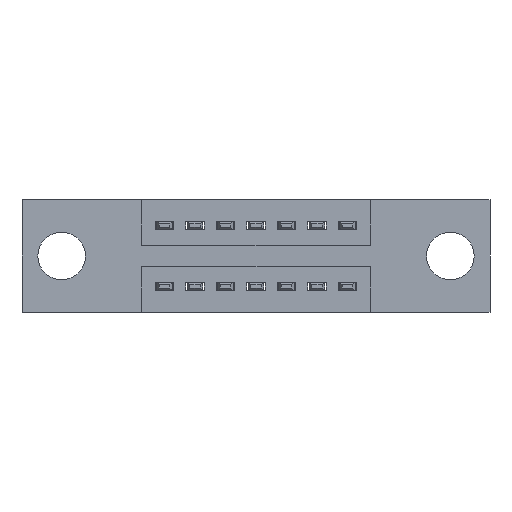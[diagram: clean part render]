
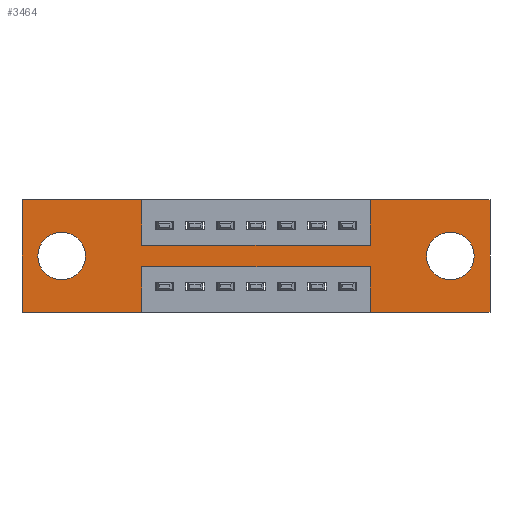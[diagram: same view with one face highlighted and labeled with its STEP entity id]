
A CAD part, front view. The second image highlights one B-rep face of the part: STEP entity #3464.
In plain terms, the highlighted planar face has unit normal (0, -1, 0).
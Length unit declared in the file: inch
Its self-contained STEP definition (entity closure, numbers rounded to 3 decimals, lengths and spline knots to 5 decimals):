
#102 = LINE ( 'NONE', #6496, #3637 ) ;
#240 = ORIENTED_EDGE ( 'NONE', *, *, #6238, .T. ) ;
#433 = CARTESIAN_POINT ( 'NONE',  ( 1.535, 0., 0. ) ) ;
#499 = EDGE_CURVE ( 'NONE', #3250, #2320, #7963, .T. ) ;
#530 = VERTEX_POINT ( 'NONE', #4773 ) ;
#573 = DIRECTION ( 'NONE',  ( 0., 1., 0. ) ) ;
#645 = CARTESIAN_POINT ( 'NONE',  ( 0., 0., -0.37 ) ) ;
#693 = ORIENTED_EDGE ( 'NONE', *, *, #1071, .F. ) ;
#815 = CARTESIAN_POINT ( 'NONE',  ( 1.535, 0., 0. ) ) ;
#839 = LINE ( 'NONE', #5701, #4201 ) ;
#951 = VECTOR ( 'NONE', #8858, 39.37008 ) ;
#953 = LINE ( 'NONE', #2516, #1004 ) ;
#1004 = VECTOR ( 'NONE', #5005, 39.37008 ) ;
#1071 = EDGE_CURVE ( 'NONE', #9457, #1078, #839, .T. ) ;
#1078 = VERTEX_POINT ( 'NONE', #6451 ) ;
#1094 = DIRECTION ( 'NONE',  ( 0., 0., 1. ) ) ;
#1287 = VERTEX_POINT ( 'NONE', #5912 ) ;
#1361 = AXIS2_PLACEMENT_3D ( 'NONE', #7787, #573, #3607 ) ;
#1465 = VERTEX_POINT ( 'NONE', #2401 ) ;
#1709 = EDGE_CURVE ( 'NONE', #1287, #2211, #2067, .T. ) ;
#1719 = AXIS2_PLACEMENT_3D ( 'NONE', #6663, #4917, #9910 ) ;
#1809 = VECTOR ( 'NONE', #9220, 39.37008 ) ;
#1819 = ORIENTED_EDGE ( 'NONE', *, *, #499, .F. ) ;
#1907 = ORIENTED_EDGE ( 'NONE', *, *, #7766, .F. ) ;
#1965 = DIRECTION ( 'NONE',  ( 0., 0., 1. ) ) ;
#1994 = ORIENTED_EDGE ( 'NONE', *, *, #2179, .F. ) ;
#2067 = LINE ( 'NONE', #6748, #8802 ) ;
#2179 = EDGE_CURVE ( 'NONE', #1465, #530, #3560, .T. ) ;
#2211 = VERTEX_POINT ( 'NONE', #7625 ) ;
#2268 = CARTESIAN_POINT ( 'NONE',  ( 1.405, 0., -0.263 ) ) ;
#2304 = EDGE_CURVE ( 'NONE', #9326, #5478, #9652, .T. ) ;
#2320 = VERTEX_POINT ( 'NONE', #7899 ) ;
#2352 = ORIENTED_EDGE ( 'NONE', *, *, #10429, .T. ) ;
#2386 = DIRECTION ( 'NONE',  ( 0., 0., -1. ) ) ;
#2401 = CARTESIAN_POINT ( 'NONE',  ( 0., 0., 0. ) ) ;
#2409 = EDGE_CURVE ( 'NONE', #9367, #4987, #10345, .T. ) ;
#2419 = DIRECTION ( 'NONE',  ( -1., 0., 0. ) ) ;
#2483 = ORIENTED_EDGE ( 'NONE', *, *, #1709, .F. ) ;
#2516 = CARTESIAN_POINT ( 'NONE',  ( 0., 0., 0. ) ) ;
#2690 = DIRECTION ( 'NONE',  ( 0., -1., 0. ) ) ;
#2788 = ORIENTED_EDGE ( 'NONE', *, *, #9125, .F. ) ;
#2797 = DIRECTION ( 'NONE',  ( 0., 0., -1. ) ) ;
#3108 = ORIENTED_EDGE ( 'NONE', *, *, #2409, .T. ) ;
#3250 = VERTEX_POINT ( 'NONE', #4840 ) ;
#3322 = VERTEX_POINT ( 'NONE', #433 ) ;
#3384 = EDGE_CURVE ( 'NONE', #4987, #9367, #4034, .T. ) ;
#3464 = ADVANCED_FACE ( 'NONE', ( #4462, #9203, #6687 ), #5891, .T. ) ;
#3549 = VECTOR ( 'NONE', #9284, 39.37008 ) ;
#3560 = LINE ( 'NONE', #9234, #3549 ) ;
#3607 = DIRECTION ( 'NONE',  ( 0., 0., 1. ) ) ;
#3637 = VECTOR ( 'NONE', #8201, 39.37008 ) ;
#3849 = CARTESIAN_POINT ( 'NONE',  ( 1.1425, 0., -0.37 ) ) ;
#4034 = CIRCLE ( 'NONE', #6555, 0.078 ) ;
#4201 = VECTOR ( 'NONE', #8101, 39.37008 ) ;
#4323 = ORIENTED_EDGE ( 'NONE', *, *, #7859, .F. ) ;
#4358 = CARTESIAN_POINT ( 'NONE',  ( 0., 0., -0.37 ) ) ;
#4414 = DIRECTION ( 'NONE',  ( 0., 1., 0. ) ) ;
#4426 = CARTESIAN_POINT ( 'NONE',  ( 0.13, 0., -0.185 ) ) ;
#4462 = FACE_BOUND ( 'NONE', #4902, .T. ) ;
#4491 = EDGE_LOOP ( 'NONE', ( #1907, #6309, #9338, #1819, #6813, #7499, #6248, #693, #2788, #1994, #4323, #2483 ) ) ;
#4658 = CARTESIAN_POINT ( 'NONE',  ( 0.3925, 0., -0.22 ) ) ;
#4773 = CARTESIAN_POINT ( 'NONE',  ( 0.3925, 0., 0. ) ) ;
#4775 = CARTESIAN_POINT ( 'NONE',  ( 1.1425, 0., -0.22 ) ) ;
#4840 = CARTESIAN_POINT ( 'NONE',  ( 1.535, 0., -0.37 ) ) ;
#4902 = EDGE_LOOP ( 'NONE', ( #5077, #3108 ) ) ;
#4917 = DIRECTION ( 'NONE',  ( 0., 1., 0. ) ) ;
#4987 = VERTEX_POINT ( 'NONE', #7512 ) ;
#5005 = DIRECTION ( 'NONE',  ( 1., 0., 0. ) ) ;
#5020 = CIRCLE ( 'NONE', #1361, 0.078 ) ;
#5055 = LINE ( 'NONE', #815, #8057 ) ;
#5077 = ORIENTED_EDGE ( 'NONE', *, *, #3384, .T. ) ;
#5270 = CARTESIAN_POINT ( 'NONE',  ( 0., 0., 0. ) ) ;
#5406 = LINE ( 'NONE', #9346, #8771 ) ;
#5478 = VERTEX_POINT ( 'NONE', #10434 ) ;
#5701 = CARTESIAN_POINT ( 'NONE',  ( 0.3925, 0., -0.15 ) ) ;
#5879 = AXIS2_PLACEMENT_3D ( 'NONE', #4358, #2690, #7688 ) ;
#5891 = PLANE ( 'NONE',  #5879 ) ;
#5908 = CARTESIAN_POINT ( 'NONE',  ( 0.13, 0., -0.263 ) ) ;
#5912 = CARTESIAN_POINT ( 'NONE',  ( 0.3925, 0., -0.37 ) ) ;
#6037 = DIRECTION ( 'NONE',  ( 0., 0., -1. ) ) ;
#6238 = EDGE_CURVE ( 'NONE', #6681, #7256, #5020, .T. ) ;
#6248 = ORIENTED_EDGE ( 'NONE', *, *, #7527, .F. ) ;
#6309 = ORIENTED_EDGE ( 'NONE', *, *, #2304, .F. ) ;
#6451 = CARTESIAN_POINT ( 'NONE',  ( 1.1425, 0., -0.15 ) ) ;
#6496 = CARTESIAN_POINT ( 'NONE',  ( 0.3925, 0., -0.37 ) ) ;
#6555 = AXIS2_PLACEMENT_3D ( 'NONE', #7535, #4414, #2797 ) ;
#6570 = CARTESIAN_POINT ( 'NONE',  ( 0.13, 0., -0.107 ) ) ;
#6663 = CARTESIAN_POINT ( 'NONE',  ( 1.405, 0., -0.185 ) ) ;
#6681 = VERTEX_POINT ( 'NONE', #5908 ) ;
#6687 = FACE_OUTER_BOUND ( 'NONE', #4491, .T. ) ;
#6748 = CARTESIAN_POINT ( 'NONE',  ( 0., 0., -0.37 ) ) ;
#6813 = ORIENTED_EDGE ( 'NONE', *, *, #8854, .F. ) ;
#6815 = LINE ( 'NONE', #5270, #1809 ) ;
#7132 = EDGE_LOOP ( 'NONE', ( #2352, #240 ) ) ;
#7256 = VERTEX_POINT ( 'NONE', #6570 ) ;
#7467 = CARTESIAN_POINT ( 'NONE',  ( 0.3925, 0., -0.15 ) ) ;
#7499 = ORIENTED_EDGE ( 'NONE', *, *, #9894, .F. ) ;
#7512 = CARTESIAN_POINT ( 'NONE',  ( 1.405, 0., -0.107 ) ) ;
#7527 = EDGE_CURVE ( 'NONE', #1078, #9092, #7953, .T. ) ;
#7535 = CARTESIAN_POINT ( 'NONE',  ( 1.405, 0., -0.185 ) ) ;
#7625 = CARTESIAN_POINT ( 'NONE',  ( 0., 0., -0.37 ) ) ;
#7688 = DIRECTION ( 'NONE',  ( 0., 0., -1. ) ) ;
#7701 = VECTOR ( 'NONE', #1094, 39.37008 ) ;
#7766 = EDGE_CURVE ( 'NONE', #5478, #1287, #102, .T. ) ;
#7787 = CARTESIAN_POINT ( 'NONE',  ( 0.13, 0., -0.185 ) ) ;
#7859 = EDGE_CURVE ( 'NONE', #2211, #1465, #6815, .T. ) ;
#7899 = CARTESIAN_POINT ( 'NONE',  ( 1.1425, 0., -0.37 ) ) ;
#7953 = LINE ( 'NONE', #9597, #951 ) ;
#7963 = LINE ( 'NONE', #645, #8252 ) ;
#8057 = VECTOR ( 'NONE', #2386, 39.37008 ) ;
#8101 = DIRECTION ( 'NONE',  ( 1., 0., 0. ) ) ;
#8201 = DIRECTION ( 'NONE',  ( 0., 0., -1. ) ) ;
#8252 = VECTOR ( 'NONE', #10379, 39.37008 ) ;
#8287 = CARTESIAN_POINT ( 'NONE',  ( 1.1425, 0., 0. ) ) ;
#8300 = AXIS2_PLACEMENT_3D ( 'NONE', #4426, #8350, #1965 ) ;
#8350 = DIRECTION ( 'NONE',  ( 0., 1., 0. ) ) ;
#8450 = VECTOR ( 'NONE', #2419, 39.37008 ) ;
#8456 = DIRECTION ( 'NONE',  ( -1., 0., 0. ) ) ;
#8771 = VECTOR ( 'NONE', #6037, 39.37008 ) ;
#8786 = EDGE_CURVE ( 'NONE', #2320, #9326, #10275, .T. ) ;
#8802 = VECTOR ( 'NONE', #8456, 39.37008 ) ;
#8825 = CIRCLE ( 'NONE', #8300, 0.078 ) ;
#8854 = EDGE_CURVE ( 'NONE', #3322, #3250, #5055, .T. ) ;
#8858 = DIRECTION ( 'NONE',  ( 0., 0., 1. ) ) ;
#9092 = VERTEX_POINT ( 'NONE', #8287 ) ;
#9125 = EDGE_CURVE ( 'NONE', #530, #9457, #5406, .T. ) ;
#9203 = FACE_BOUND ( 'NONE', #7132, .T. ) ;
#9220 = DIRECTION ( 'NONE',  ( 0., 0., 1. ) ) ;
#9234 = CARTESIAN_POINT ( 'NONE',  ( 0., 0., 0. ) ) ;
#9284 = DIRECTION ( 'NONE',  ( 1., 0., 0. ) ) ;
#9326 = VERTEX_POINT ( 'NONE', #4775 ) ;
#9338 = ORIENTED_EDGE ( 'NONE', *, *, #8786, .F. ) ;
#9346 = CARTESIAN_POINT ( 'NONE',  ( 0.3925, 0., 0. ) ) ;
#9367 = VERTEX_POINT ( 'NONE', #2268 ) ;
#9457 = VERTEX_POINT ( 'NONE', #7467 ) ;
#9597 = CARTESIAN_POINT ( 'NONE',  ( 1.1425, 0., 0. ) ) ;
#9652 = LINE ( 'NONE', #4658, #8450 ) ;
#9894 = EDGE_CURVE ( 'NONE', #9092, #3322, #953, .T. ) ;
#9910 = DIRECTION ( 'NONE',  ( 0., 0., -1. ) ) ;
#10275 = LINE ( 'NONE', #3849, #7701 ) ;
#10345 = CIRCLE ( 'NONE', #1719, 0.078 ) ;
#10379 = DIRECTION ( 'NONE',  ( -1., 0., 0. ) ) ;
#10429 = EDGE_CURVE ( 'NONE', #7256, #6681, #8825, .T. ) ;
#10434 = CARTESIAN_POINT ( 'NONE',  ( 0.3925, 0., -0.22 ) ) ;
